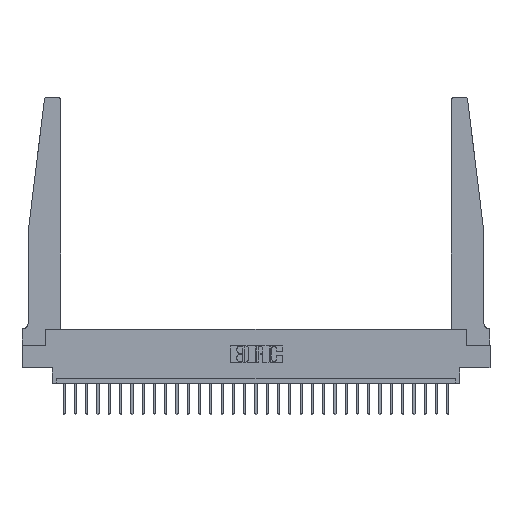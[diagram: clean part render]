
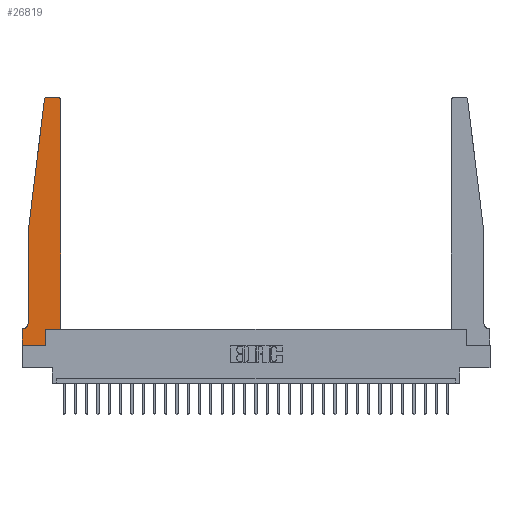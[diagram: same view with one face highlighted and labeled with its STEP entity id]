
A CAD part, top view. The second image highlights one B-rep face of the part: STEP entity #26819.
In plain terms, the highlighted planar face has unit normal (0, 0, 1).
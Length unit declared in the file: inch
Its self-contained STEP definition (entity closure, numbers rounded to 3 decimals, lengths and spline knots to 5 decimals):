
#21 = CARTESIAN_POINT ( 'NONE',  ( 0.25, 2.75, 0.37 ) ) ;
#30 = VECTOR ( 'NONE', #230, 39.37008 ) ;
#149 = EDGE_CURVE ( 'NONE', #1061, #27241, #2507, .T. ) ;
#158 = DIRECTION ( 'NONE',  ( 1., 0., 0. ) ) ;
#230 = DIRECTION ( 'NONE',  ( -0.122, -0.992, 0. ) ) ;
#432 = DIRECTION ( 'NONE',  ( 0., -1., 0. ) ) ;
#452 = CARTESIAN_POINT ( 'NONE',  ( 0.24675, 2.72367, 0.37 ) ) ;
#641 = CARTESIAN_POINT ( 'NONE',  ( 0.27653, 2.75, 0.37 ) ) ;
#1061 = VERTEX_POINT ( 'NONE', #641 ) ;
#1097 = EDGE_CURVE ( 'NONE', #19652, #5348, #13404, .T. ) ;
#1915 = ORIENTED_EDGE ( 'NONE', *, *, #1097, .T. ) ;
#2507 = CIRCLE ( 'NONE', #27505, 0.03 ) ;
#2730 = VERTEX_POINT ( 'NONE', #21671 ) ;
#3453 = CARTESIAN_POINT ( 'NONE',  ( 0.065, 1.25, 0.37 ) ) ;
#3787 = ORIENTED_EDGE ( 'NONE', *, *, #10385, .T. ) ;
#4362 = AXIS2_PLACEMENT_3D ( 'NONE', #22607, #11803, #26797 ) ;
#4599 = EDGE_CURVE ( 'NONE', #25624, #6489, #21834, .T. ) ;
#5000 = VECTOR ( 'NONE', #14936, 39.37008 ) ;
#5348 = VERTEX_POINT ( 'NONE', #16223 ) ;
#5461 = CARTESIAN_POINT ( 'NONE',  ( 0.065, 0.2375, 0.37 ) ) ;
#5676 = DIRECTION ( 'NONE',  ( 0., -1., 0. ) ) ;
#5680 = CARTESIAN_POINT ( 'NONE',  ( 0.425, 0.18, 0.37 ) ) ;
#5820 = CARTESIAN_POINT ( 'NONE',  ( 0.2605, 0.18, 0.37 ) ) ;
#5923 = ORIENTED_EDGE ( 'NONE', *, *, #12208, .T. ) ;
#6489 = VERTEX_POINT ( 'NONE', #17317 ) ;
#6804 = ORIENTED_EDGE ( 'NONE', *, *, #25833, .T. ) ;
#7063 = ORIENTED_EDGE ( 'NONE', *, *, #16823, .T. ) ;
#7417 = CARTESIAN_POINT ( 'NONE',  ( 0.2605, 0., 0.37 ) ) ;
#8348 = CARTESIAN_POINT ( 'NONE',  ( 0.065, 0.1875, 0.37 ) ) ;
#9033 = CARTESIAN_POINT ( 'NONE',  ( 0.395, 2.72, 0.37 ) ) ;
#9110 = ORIENTED_EDGE ( 'NONE', *, *, #10839, .T. ) ;
#9120 = CARTESIAN_POINT ( 'NONE',  ( 0., 0., 0.37 ) ) ;
#9326 = VERTEX_POINT ( 'NONE', #24633 ) ;
#9367 = ORIENTED_EDGE ( 'NONE', *, *, #4599, .T. ) ;
#9644 = VERTEX_POINT ( 'NONE', #5680 ) ;
#9807 = VECTOR ( 'NONE', #158, 39.37008 ) ;
#10385 = EDGE_CURVE ( 'NONE', #6489, #25201, #15225, .T. ) ;
#10457 = CARTESIAN_POINT ( 'NONE',  ( 0.065, 1.25, 0.37 ) ) ;
#10561 = EDGE_CURVE ( 'NONE', #9644, #24450, #12207, .T. ) ;
#10839 = EDGE_CURVE ( 'NONE', #25201, #2730, #19507, .T. ) ;
#11245 = DIRECTION ( 'NONE',  ( 1., 0., 0. ) ) ;
#11349 = DIRECTION ( 'NONE',  ( 0., 0., 1. ) ) ;
#11516 = VECTOR ( 'NONE', #432, 39.37008 ) ;
#11599 = FACE_OUTER_BOUND ( 'NONE', #20335, .T. ) ;
#11803 = DIRECTION ( 'NONE',  ( 0., 0., 1. ) ) ;
#11898 = PLANE ( 'NONE',  #4362 ) ;
#11909 = EDGE_CURVE ( 'NONE', #2730, #19652, #18291, .T. ) ;
#12207 = LINE ( 'NONE', #25116, #17183 ) ;
#12208 = EDGE_CURVE ( 'NONE', #9326, #25624, #16299, .T. ) ;
#13228 = ORIENTED_EDGE ( 'NONE', *, *, #149, .T. ) ;
#13404 = LINE ( 'NONE', #5820, #25440 ) ;
#13552 = ORIENTED_EDGE ( 'NONE', *, *, #18675, .T. ) ;
#13981 = VECTOR ( 'NONE', #5676, 39.37008 ) ;
#14339 = LINE ( 'NONE', #10457, #30 ) ;
#14367 = AXIS2_PLACEMENT_3D ( 'NONE', #9033, #11349, #11245 ) ;
#14936 = DIRECTION ( 'NONE',  ( -1., 0., 0. ) ) ;
#15225 = LINE ( 'NONE', #8348, #20873 ) ;
#15835 = LINE ( 'NONE', #19308, #9807 ) ;
#16223 = CARTESIAN_POINT ( 'NONE',  ( 0.2605, 0.18, 0.37 ) ) ;
#16299 = LINE ( 'NONE', #3453, #13981 ) ;
#16823 = EDGE_CURVE ( 'NONE', #24450, #16953, #17386, .T. ) ;
#16953 = VERTEX_POINT ( 'NONE', #24035 ) ;
#17183 = VECTOR ( 'NONE', #27246, 39.37008 ) ;
#17317 = CARTESIAN_POINT ( 'NONE',  ( 0.015, 0.1875, 0.37 ) ) ;
#17386 = CIRCLE ( 'NONE', #14367, 0.03 ) ;
#17722 = ORIENTED_EDGE ( 'NONE', *, *, #22194, .T. ) ;
#18291 = LINE ( 'NONE', #9120, #25645 ) ;
#18630 = DIRECTION ( 'NONE',  ( 0., 1., 0. ) ) ;
#18675 = EDGE_CURVE ( 'NONE', #16953, #1061, #20639, .T. ) ;
#18770 = ORIENTED_EDGE ( 'NONE', *, *, #10561, .T. ) ;
#19052 = CARTESIAN_POINT ( 'NONE',  ( 0., 0.1875, 0.37 ) ) ;
#19302 = DIRECTION ( 'NONE',  ( 1., 0., 0. ) ) ;
#19308 = CARTESIAN_POINT ( 'NONE',  ( 0.425, 0.18, 0.37 ) ) ;
#19507 = LINE ( 'NONE', #24063, #11516 ) ;
#19578 = CARTESIAN_POINT ( 'NONE',  ( 0.27653, 2.72, 0.37 ) ) ;
#19652 = VERTEX_POINT ( 'NONE', #7417 ) ;
#20335 = EDGE_LOOP ( 'NONE', ( #13552, #13228, #6804, #5923, #9367, #3787, #9110, #26391, #1915, #17722, #18770, #7063 ) ) ;
#20639 = LINE ( 'NONE', #21, #5000 ) ;
#20873 = VECTOR ( 'NONE', #23248, 39.37008 ) ;
#20878 = DIRECTION ( 'NONE',  ( 0., 0., -1. ) ) ;
#21671 = CARTESIAN_POINT ( 'NONE',  ( 0., 0., 0.37 ) ) ;
#21834 = CIRCLE ( 'NONE', #27381, 0.05 ) ;
#22194 = EDGE_CURVE ( 'NONE', #5348, #9644, #15835, .T. ) ;
#22607 = CARTESIAN_POINT ( 'NONE',  ( 0., 0.1875, 0.37 ) ) ;
#22920 = CARTESIAN_POINT ( 'NONE',  ( 0.015, 0.2375, 0.37 ) ) ;
#23015 = DIRECTION ( 'NONE',  ( -1., 0., 0. ) ) ;
#23248 = DIRECTION ( 'NONE',  ( -1., 0., 0. ) ) ;
#23874 = DIRECTION ( 'NONE',  ( 0., 0., 1. ) ) ;
#24035 = CARTESIAN_POINT ( 'NONE',  ( 0.395, 2.75, 0.37 ) ) ;
#24063 = CARTESIAN_POINT ( 'NONE',  ( 0., 0., 0.37 ) ) ;
#24120 = DIRECTION ( 'NONE',  ( 1., 0., 0. ) ) ;
#24450 = VERTEX_POINT ( 'NONE', #25357 ) ;
#24633 = CARTESIAN_POINT ( 'NONE',  ( 0.065, 1.25, 0.37 ) ) ;
#25116 = CARTESIAN_POINT ( 'NONE',  ( 0.425, 0.18, 0.37 ) ) ;
#25201 = VERTEX_POINT ( 'NONE', #19052 ) ;
#25357 = CARTESIAN_POINT ( 'NONE',  ( 0.425, 2.72, 0.37 ) ) ;
#25440 = VECTOR ( 'NONE', #18630, 39.37008 ) ;
#25624 = VERTEX_POINT ( 'NONE', #5461 ) ;
#25645 = VECTOR ( 'NONE', #24120, 39.37008 ) ;
#25833 = EDGE_CURVE ( 'NONE', #27241, #9326, #14339, .T. ) ;
#26391 = ORIENTED_EDGE ( 'NONE', *, *, #11909, .T. ) ;
#26797 = DIRECTION ( 'NONE',  ( 1., 0., 0. ) ) ;
#26819 = ADVANCED_FACE ( 'NONE', ( #11599 ), #11898, .T. ) ;
#27241 = VERTEX_POINT ( 'NONE', #452 ) ;
#27246 = DIRECTION ( 'NONE',  ( 0., 1., 0. ) ) ;
#27381 = AXIS2_PLACEMENT_3D ( 'NONE', #22920, #20878, #23015 ) ;
#27505 = AXIS2_PLACEMENT_3D ( 'NONE', #19578, #23874, #19302 ) ;
